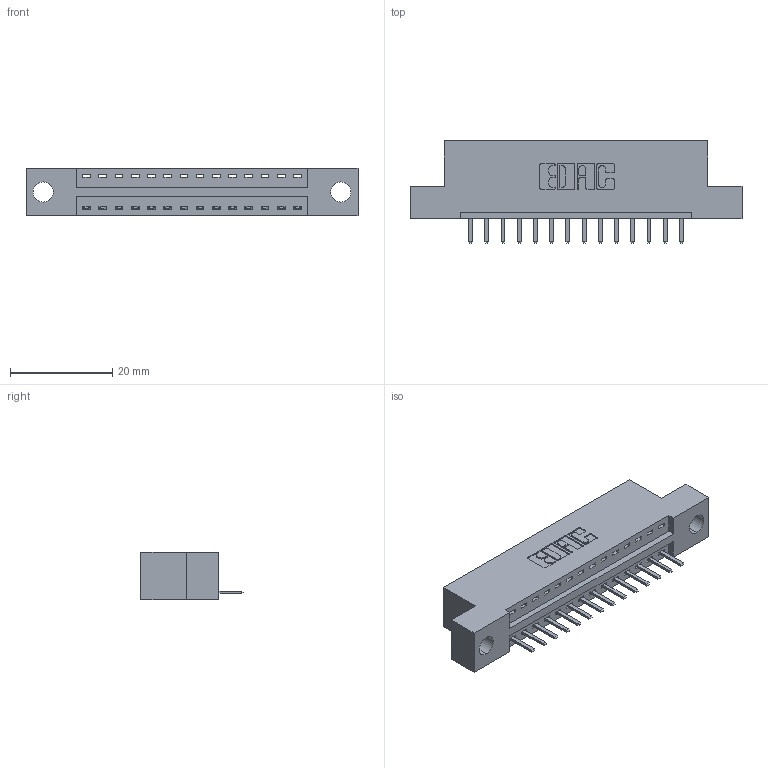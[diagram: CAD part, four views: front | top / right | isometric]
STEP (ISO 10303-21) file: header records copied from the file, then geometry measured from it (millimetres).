
FILE_DESCRIPTION (( 'STEP AP203' ), '1' );
FILE_NAME ('396-014-520-104.STEP', '2019-10-26T16:28:53', ( '' ), ( '' ), 'SwSTEP 2.0', 'SolidWorks 2016', '' );
FILE_SCHEMA (( 'CONFIG_CONTROL_DESIGN' ));
Length unit declared in the file: inch
Products named in the file (3): 396-014-520-104; 346 Part_Flush Mounting Lugs - 0.156 Dia-TH; 345-292-001_345-293-120
Assembly tree (15 placements, depth 2):
  396-014-520-104
    346 Part_Flush Mounting Lugs - 0.156 Dia-TH
    345-292-001_345-293-120  x14
Bounding box: 65.02 x 20.02 x 9.4 mm (x, y, z)
Volume: 5903.2 mm3; surface area: 6746.6 mm2
Topology: 15 solids, 15 shells, 990 faces, 2905 edges, 1898 vertices
Faces by surface type: plane 664, cylinder 326
Entity records: 12575 total; most frequent: CARTESIAN_POINT 2182, ORIENTED_EDGE 2118, DIRECTION 1947, EDGE_CURVE 1059, VECTOR 867, LINE 867, VERTEX_POINT 702, AXIS2_PLACEMENT_3D 540
